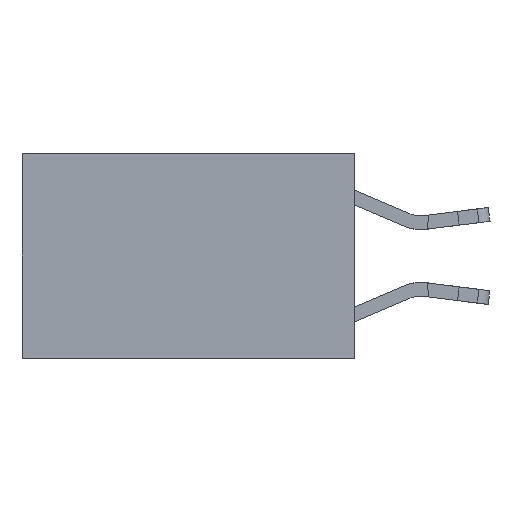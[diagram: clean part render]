
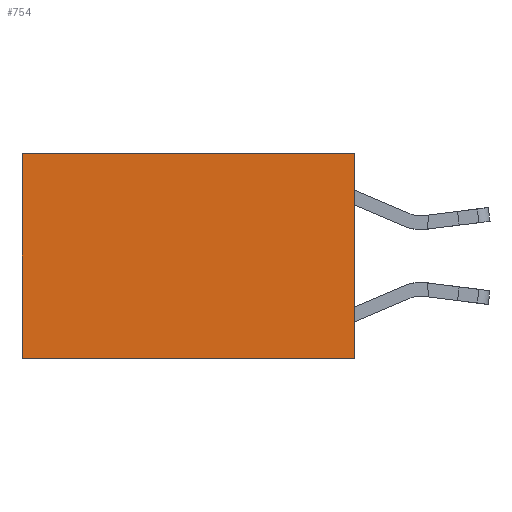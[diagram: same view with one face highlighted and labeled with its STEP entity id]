
A CAD part, left-side view. The second image highlights one B-rep face of the part: STEP entity #754.
In plain terms, the highlighted planar face has unit normal (-1, 0, 0).
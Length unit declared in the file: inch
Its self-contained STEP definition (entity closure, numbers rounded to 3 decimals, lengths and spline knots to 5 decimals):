
#672 = CARTESIAN_POINT ( 'NONE',  ( 0.2625, 0., 0. ) ) ;
#754 = ADVANCED_FACE ( 'NONE', ( #10702 ), #13498, .F. ) ;
#1136 = VECTOR ( 'NONE', #8331, 39.37008 ) ;
#1143 = DIRECTION ( 'NONE',  ( 0., 1., 0. ) ) ;
#1302 = CARTESIAN_POINT ( 'NONE',  ( 0.2625, 0.6, 0. ) ) ;
#1671 = EDGE_LOOP ( 'NONE', ( #3759, #6970, #6478, #3383 ) ) ;
#1711 = LINE ( 'NONE', #4737, #8682 ) ;
#1905 = VERTEX_POINT ( 'NONE', #5595 ) ;
#1981 = DIRECTION ( 'NONE',  ( 0., 0., -1. ) ) ;
#3383 = ORIENTED_EDGE ( 'NONE', *, *, #14553, .T. ) ;
#3489 = AXIS2_PLACEMENT_3D ( 'NONE', #672, #11428, #14353 ) ;
#3759 = ORIENTED_EDGE ( 'NONE', *, *, #5846, .T. ) ;
#3818 = LINE ( 'NONE', #10698, #14302 ) ;
#4312 = EDGE_CURVE ( 'NONE', #15172, #1905, #3818, .T. ) ;
#4702 = CARTESIAN_POINT ( 'NONE',  ( 0.2625, 0., 0. ) ) ;
#4737 = CARTESIAN_POINT ( 'NONE',  ( 0.2625, 0., 0. ) ) ;
#4894 = LINE ( 'NONE', #1302, #1136 ) ;
#5015 = VERTEX_POINT ( 'NONE', #11736 ) ;
#5595 = CARTESIAN_POINT ( 'NONE',  ( 0.2625, 0.6, -0.37 ) ) ;
#5846 = EDGE_CURVE ( 'NONE', #12423, #1905, #4894, .T. ) ;
#6133 = DIRECTION ( 'NONE',  ( 0., 1., 0. ) ) ;
#6478 = ORIENTED_EDGE ( 'NONE', *, *, #17306, .F. ) ;
#6640 = VECTOR ( 'NONE', #6133, 39.37008 ) ;
#6970 = ORIENTED_EDGE ( 'NONE', *, *, #4312, .F. ) ;
#8331 = DIRECTION ( 'NONE',  ( 0., 0., -1. ) ) ;
#8682 = VECTOR ( 'NONE', #1981, 39.37008 ) ;
#8990 = CARTESIAN_POINT ( 'NONE',  ( 0.2625, 0.6, 0. ) ) ;
#10698 = CARTESIAN_POINT ( 'NONE',  ( 0.2625, 0., -0.37 ) ) ;
#10702 = FACE_OUTER_BOUND ( 'NONE', #1671, .T. ) ;
#11428 = DIRECTION ( 'NONE',  ( 1., 0., 0. ) ) ;
#11736 = CARTESIAN_POINT ( 'NONE',  ( 0.2625, 0., 0. ) ) ;
#12423 = VERTEX_POINT ( 'NONE', #8990 ) ;
#12837 = CARTESIAN_POINT ( 'NONE',  ( 0.2625, 0., -0.37 ) ) ;
#13498 = PLANE ( 'NONE',  #3489 ) ;
#14252 = LINE ( 'NONE', #4702, #6640 ) ;
#14302 = VECTOR ( 'NONE', #1143, 39.37008 ) ;
#14353 = DIRECTION ( 'NONE',  ( 0., 0., -1. ) ) ;
#14553 = EDGE_CURVE ( 'NONE', #5015, #12423, #14252, .T. ) ;
#15172 = VERTEX_POINT ( 'NONE', #12837 ) ;
#17306 = EDGE_CURVE ( 'NONE', #5015, #15172, #1711, .T. ) ;
